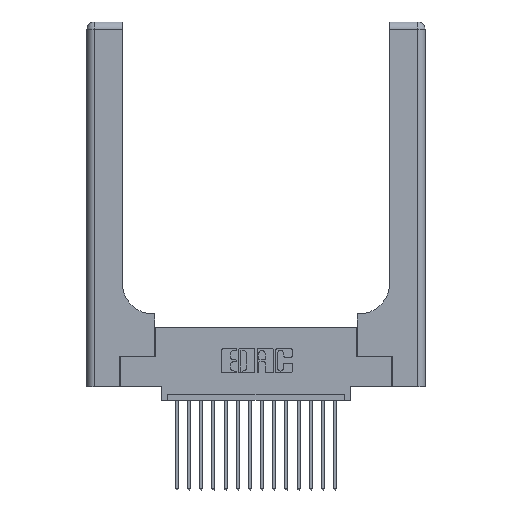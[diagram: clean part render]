
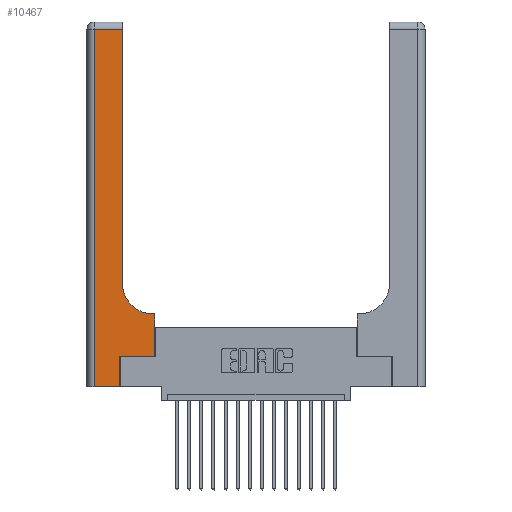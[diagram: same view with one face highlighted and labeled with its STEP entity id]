
A CAD part, top view. The second image highlights one B-rep face of the part: STEP entity #10467.
In plain terms, the highlighted planar face has unit normal (0, 0, 1).
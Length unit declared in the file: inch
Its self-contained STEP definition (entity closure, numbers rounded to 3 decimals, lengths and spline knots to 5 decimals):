
#447 = ORIENTED_EDGE ( 'NONE', *, *, #799, .T. ) ;
#456 = DIRECTION ( 'NONE',  ( -1., 0., 0. ) ) ;
#522 = LINE ( 'NONE', #17002, #5264 ) ;
#720 = CARTESIAN_POINT ( 'NONE',  ( 0.2915, 2.94, 0.37 ) ) ;
#759 = CARTESIAN_POINT ( 'NONE',  ( 0.06, 2.94, 0.37 ) ) ;
#799 = EDGE_CURVE ( 'NONE', #15221, #12346, #875, .T. ) ;
#866 = DIRECTION ( 'NONE',  ( 1., 0., 0. ) ) ;
#875 = LINE ( 'NONE', #14063, #10579 ) ;
#1248 = LINE ( 'NONE', #18439, #10465 ) ;
#1363 = LINE ( 'NONE', #4829, #8926 ) ;
#1901 = DIRECTION ( 'NONE',  ( -1., 0., 0. ) ) ;
#2248 = ORIENTED_EDGE ( 'NONE', *, *, #6404, .T. ) ;
#2386 = CARTESIAN_POINT ( 'NONE',  ( 0., 0., 0.37 ) ) ;
#2832 = VERTEX_POINT ( 'NONE', #19421 ) ;
#3001 = DIRECTION ( 'NONE',  ( 0., 0., -1. ) ) ;
#3161 = CARTESIAN_POINT ( 'NONE',  ( 0., 3., 0.37 ) ) ;
#3699 = AXIS2_PLACEMENT_3D ( 'NONE', #10475, #3001, #9081 ) ;
#4252 = EDGE_CURVE ( 'NONE', #15623, #15435, #522, .T. ) ;
#4503 = CARTESIAN_POINT ( 'NONE',  ( 0.5585, 0.6, 0.37 ) ) ;
#4633 = ORIENTED_EDGE ( 'NONE', *, *, #5550, .T. ) ;
#4787 = CARTESIAN_POINT ( 'NONE',  ( 0.06, 0., 0.37 ) ) ;
#4811 = PLANE ( 'NONE',  #13918 ) ;
#4829 = CARTESIAN_POINT ( 'NONE',  ( 0., 2.94, 0.37 ) ) ;
#4841 = DIRECTION ( 'NONE',  ( -1., 0., 0. ) ) ;
#5010 = ORIENTED_EDGE ( 'NONE', *, *, #12492, .T. ) ;
#5121 = LINE ( 'NONE', #14209, #8193 ) ;
#5264 = VECTOR ( 'NONE', #6362, 39.37008 ) ;
#5480 = CARTESIAN_POINT ( 'NONE',  ( 0.2915, 0.85, 0.37 ) ) ;
#5550 = EDGE_CURVE ( 'NONE', #2832, #15623, #6358, .T. ) ;
#5609 = VERTEX_POINT ( 'NONE', #4787 ) ;
#5742 = CARTESIAN_POINT ( 'NONE',  ( 0.269, 0.25, 0.37 ) ) ;
#5884 = VERTEX_POINT ( 'NONE', #5742 ) ;
#6358 = CIRCLE ( 'NONE', #3699, 0.25 ) ;
#6362 = DIRECTION ( 'NONE',  ( 0., 1., 0. ) ) ;
#6404 = EDGE_CURVE ( 'NONE', #5609, #16044, #8229, .T. ) ;
#6586 = VECTOR ( 'NONE', #866, 39.37008 ) ;
#6657 = DIRECTION ( 'NONE',  ( 0., 0., -1. ) ) ;
#6807 = EDGE_CURVE ( 'NONE', #15435, #16498, #1363, .T. ) ;
#6822 = DIRECTION ( 'NONE',  ( 0., 1., 0. ) ) ;
#6942 = ORIENTED_EDGE ( 'NONE', *, *, #9447, .T. ) ;
#7427 = EDGE_CURVE ( 'NONE', #5884, #15221, #5121, .T. ) ;
#7765 = CARTESIAN_POINT ( 'NONE',  ( 0.269, 0., 0.37 ) ) ;
#7957 = DIRECTION ( 'NONE',  ( 0., 1., 0. ) ) ;
#8193 = VECTOR ( 'NONE', #14271, 39.37008 ) ;
#8229 = LINE ( 'NONE', #2386, #6586 ) ;
#8926 = VECTOR ( 'NONE', #456, 39.37008 ) ;
#9081 = DIRECTION ( 'NONE',  ( 1., 0., 0. ) ) ;
#9114 = EDGE_LOOP ( 'NONE', ( #9739, #12646, #13274, #2248, #5010, #10701, #447, #6942, #4633 ) ) ;
#9447 = EDGE_CURVE ( 'NONE', #12346, #2832, #1248, .T. ) ;
#9739 = ORIENTED_EDGE ( 'NONE', *, *, #4252, .T. ) ;
#10447 = CARTESIAN_POINT ( 'NONE',  ( 0.5585, 0.25, 0.37 ) ) ;
#10465 = VECTOR ( 'NONE', #4841, 39.37008 ) ;
#10467 = ADVANCED_FACE ( 'NONE', ( #11376 ), #4811, .F. ) ;
#10475 = CARTESIAN_POINT ( 'NONE',  ( 0.5415, 0.85, 0.37 ) ) ;
#10579 = VECTOR ( 'NONE', #7957, 39.37008 ) ;
#10682 = CARTESIAN_POINT ( 'NONE',  ( 0.06, 3., 0.37 ) ) ;
#10701 = ORIENTED_EDGE ( 'NONE', *, *, #7427, .T. ) ;
#11376 = FACE_OUTER_BOUND ( 'NONE', #9114, .T. ) ;
#11436 = LINE ( 'NONE', #10682, #18367 ) ;
#12346 = VERTEX_POINT ( 'NONE', #4503 ) ;
#12492 = EDGE_CURVE ( 'NONE', #16044, #5884, #18645, .T. ) ;
#12646 = ORIENTED_EDGE ( 'NONE', *, *, #6807, .T. ) ;
#13274 = ORIENTED_EDGE ( 'NONE', *, *, #13662, .T. ) ;
#13662 = EDGE_CURVE ( 'NONE', #16498, #5609, #11436, .T. ) ;
#13893 = VECTOR ( 'NONE', #6822, 39.37008 ) ;
#13918 = AXIS2_PLACEMENT_3D ( 'NONE', #3161, #6657, #1901 ) ;
#14063 = CARTESIAN_POINT ( 'NONE',  ( 0.5585, 0.25, 0.37 ) ) ;
#14209 = CARTESIAN_POINT ( 'NONE',  ( 0.269, 0.25, 0.37 ) ) ;
#14271 = DIRECTION ( 'NONE',  ( 1., 0., 0. ) ) ;
#14775 = CARTESIAN_POINT ( 'NONE',  ( 0.269, 0., 0.37 ) ) ;
#15221 = VERTEX_POINT ( 'NONE', #10447 ) ;
#15277 = DIRECTION ( 'NONE',  ( 0., -1., 0. ) ) ;
#15435 = VERTEX_POINT ( 'NONE', #720 ) ;
#15623 = VERTEX_POINT ( 'NONE', #5480 ) ;
#16044 = VERTEX_POINT ( 'NONE', #14775 ) ;
#16498 = VERTEX_POINT ( 'NONE', #759 ) ;
#17002 = CARTESIAN_POINT ( 'NONE',  ( 0.2915, 3., 0.37 ) ) ;
#18367 = VECTOR ( 'NONE', #15277, 39.37008 ) ;
#18439 = CARTESIAN_POINT ( 'NONE',  ( 0.2915, 0.6, 0.37 ) ) ;
#18645 = LINE ( 'NONE', #7765, #13893 ) ;
#19421 = CARTESIAN_POINT ( 'NONE',  ( 0.5415, 0.6, 0.37 ) ) ;
